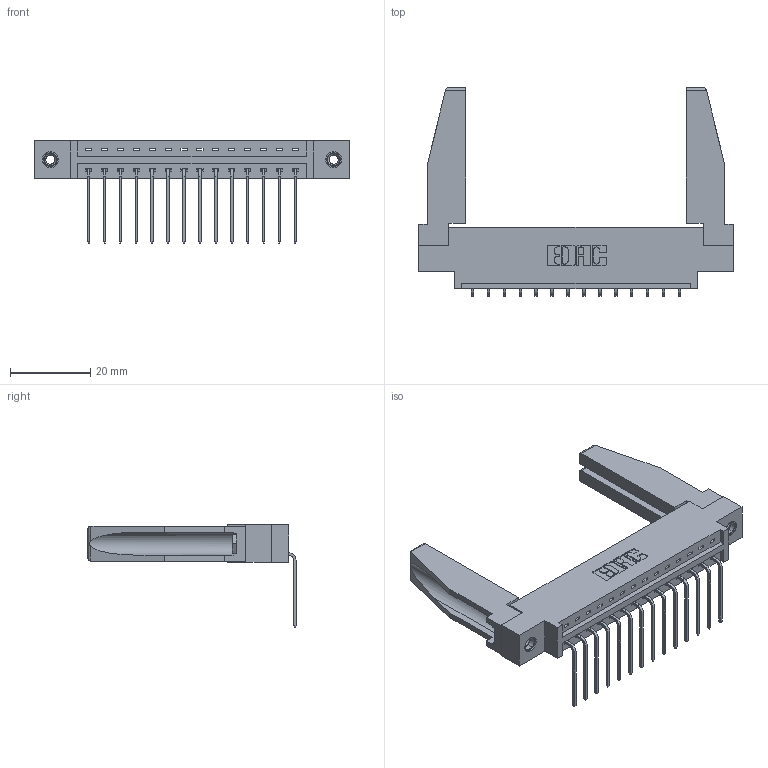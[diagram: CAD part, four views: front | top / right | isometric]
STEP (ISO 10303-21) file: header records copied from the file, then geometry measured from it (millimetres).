
FILE_DESCRIPTION (( 'STEP AP203' ), '1' );
FILE_NAME ('387-014-559-678.STEP', '2019-10-02T16:10:59', ( '' ), ( '' ), 'SwSTEP 2.0', 'SolidWorks 2016', '' );
FILE_SCHEMA (( 'CONFIG_CONTROL_DESIGN' ));
Length unit declared in the file: inch
Products named in the file (5): 307-220-078; 387-014-559-678; 345-250-001_345-250-001-102; 345-292-001_558 559 Tail - 1; 337 Part_0.170 Offset - 0.156 Dia-TI
Assembly tree (19 placements, depth 2):
  387-014-559-678
    337 Part_0.170 Offset - 0.156 Dia-TI
    345-292-001_558 559 Tail - 1  x14
    345-250-001_345-250-001-102  x2
    307-220-078  x2
Bounding box: 78.49 x 51.88 x 25.53 mm (x, y, z)
Volume: 11729.4 mm3; surface area: 12058.5 mm2
Topology: 19 solids, 19 shells, 1144 faces, 3369 edges, 2218 vertices
Faces by surface type: plane 830, cylinder 298, cone 12, torus 4
Entity records: 16684 total; most frequent: CARTESIAN_POINT 2898, ORIENTED_EDGE 2804, DIRECTION 2506, EDGE_CURVE 1402, VECTOR 1236, LINE 1236, VERTEX_POINT 928, AXIS2_PLACEMENT_3D 635
